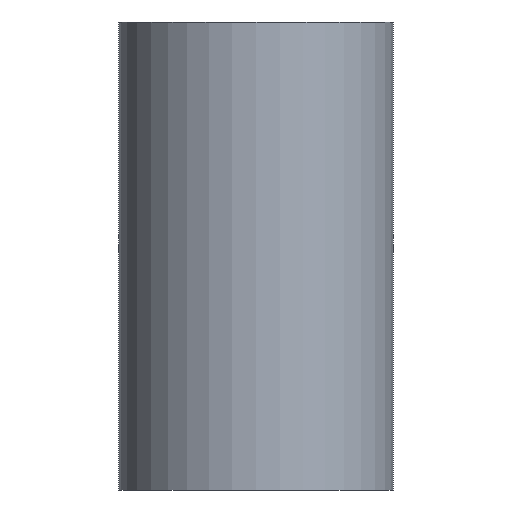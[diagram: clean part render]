
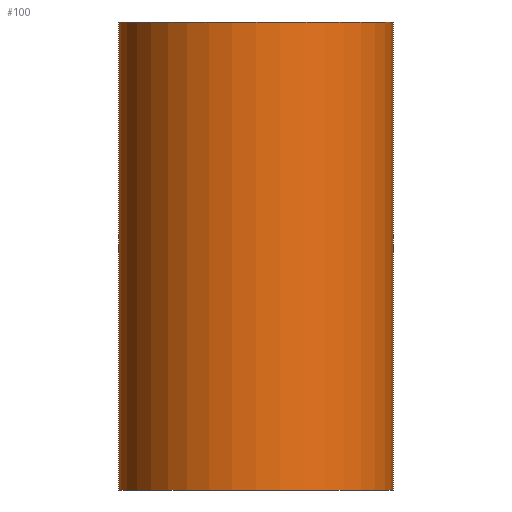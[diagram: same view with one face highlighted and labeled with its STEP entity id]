
A CAD part, front view. The second image highlights one B-rep face of the part: STEP entity #100.
In plain terms, the highlighted cylindrical face has radius 2.3 mm (diameter 4.6 mm), a full revolution.
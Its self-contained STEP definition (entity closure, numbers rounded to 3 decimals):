
#20=LINE('',#193,#22);
#22=VECTOR('',#166,2.3);
#24=CYLINDRICAL_SURFACE('',#130,2.3);
#30=FACE_OUTER_BOUND('',#38,.T.);
#38=EDGE_LOOP('',(#89,#90,#91,#92));
#45=CIRCLE('',#124,2.3);
#48=CIRCLE('',#129,2.3);
#54=VERTEX_POINT('',#183);
#56=VERTEX_POINT('',#190);
#64=EDGE_CURVE('',#54,#54,#45,.T.);
#67=EDGE_CURVE('',#56,#56,#48,.T.);
#68=EDGE_CURVE('',#56,#54,#20,.T.);
#89=ORIENTED_EDGE('',*,*,#67,.F.);
#90=ORIENTED_EDGE('',*,*,#68,.T.);
#91=ORIENTED_EDGE('',*,*,#64,.T.);
#92=ORIENTED_EDGE('',*,*,#68,.F.);
#100=ADVANCED_FACE('',(#30),#24,.T.);
#124=AXIS2_PLACEMENT_3D('',#184,#152,#153);
#129=AXIS2_PLACEMENT_3D('',#191,#162,#163);
#130=AXIS2_PLACEMENT_3D('',#192,#164,#165);
#152=DIRECTION('center_axis',(0.,0.,1.));
#153=DIRECTION('ref_axis',(1.,0.,0.));
#162=DIRECTION('center_axis',(0.,0.,1.));
#163=DIRECTION('ref_axis',(1.,0.,0.));
#164=DIRECTION('center_axis',(0.,0.,1.));
#165=DIRECTION('ref_axis',(1.,0.,0.));
#166=DIRECTION('',(0.,0.,-1.));
#183=CARTESIAN_POINT('',(7.7,10.,0.));
#184=CARTESIAN_POINT('Origin',(10.,10.,0.));
#190=CARTESIAN_POINT('',(7.7,10.,7.85));
#191=CARTESIAN_POINT('Origin',(10.,10.,7.85));
#192=CARTESIAN_POINT('Origin',(10.,10.,0.));
#193=CARTESIAN_POINT('',(7.7,10.,0.));
